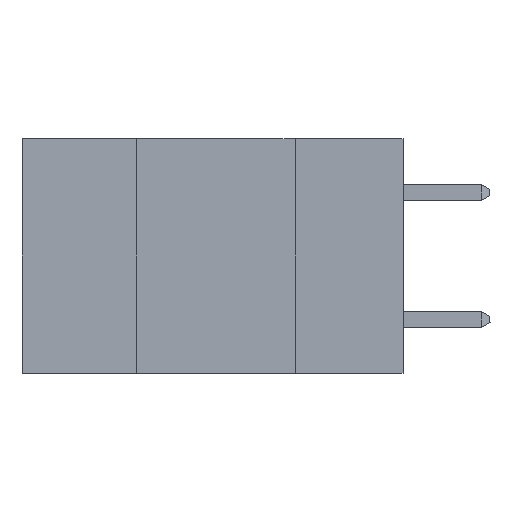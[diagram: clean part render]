
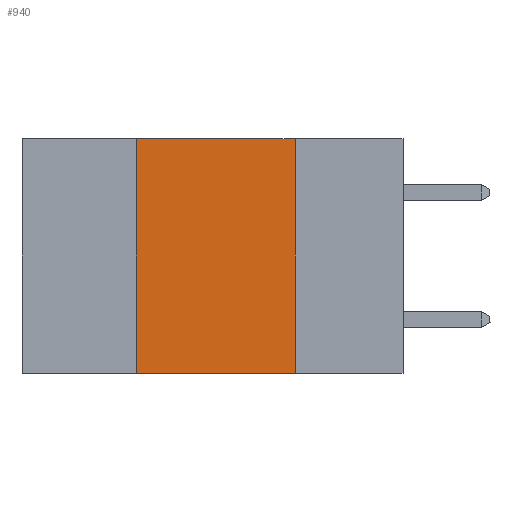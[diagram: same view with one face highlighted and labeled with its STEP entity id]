
A CAD part, left-side view. The second image highlights one B-rep face of the part: STEP entity #940.
In plain terms, the highlighted planar face has unit normal (-1, 0, 0).
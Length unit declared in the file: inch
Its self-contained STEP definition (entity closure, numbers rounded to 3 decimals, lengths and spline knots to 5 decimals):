
#160 = ORIENTED_EDGE ( 'NONE', *, *, #24087, .F. ) ;
#666 = CARTESIAN_POINT ( 'NONE',  ( 0., 0.17, 0. ) ) ;
#940 = ADVANCED_FACE ( 'NONE', ( #27256 ), #1410, .F. ) ;
#1410 = PLANE ( 'NONE',  #10255 ) ;
#1800 = VECTOR ( 'NONE', #24428, 39.37008 ) ;
#1870 = VERTEX_POINT ( 'NONE', #23510 ) ;
#2463 = EDGE_CURVE ( 'NONE', #1870, #14427, #19160, .T. ) ;
#2764 = DIRECTION ( 'NONE',  ( 0., 0., 1. ) ) ;
#2925 = CARTESIAN_POINT ( 'NONE',  ( 0., 0.6, -0.37 ) ) ;
#3157 = LINE ( 'NONE', #17607, #1800 ) ;
#4084 = VECTOR ( 'NONE', #2764, 39.37008 ) ;
#6897 = ORIENTED_EDGE ( 'NONE', *, *, #16684, .F. ) ;
#7790 = ORIENTED_EDGE ( 'NONE', *, *, #2463, .F. ) ;
#9384 = DIRECTION ( 'NONE',  ( 0., -1., 0. ) ) ;
#10255 = AXIS2_PLACEMENT_3D ( 'NONE', #12144, #12056, #14170 ) ;
#10950 = VECTOR ( 'NONE', #19508, 39.37008 ) ;
#11149 = EDGE_LOOP ( 'NONE', ( #6897, #160, #7790, #22038 ) ) ;
#11459 = VECTOR ( 'NONE', #9384, 39.37008 ) ;
#12056 = DIRECTION ( 'NONE',  ( 1., 0., 0. ) ) ;
#12144 = CARTESIAN_POINT ( 'NONE',  ( 0., 0.6, 0. ) ) ;
#13523 = VERTEX_POINT ( 'NONE', #666 ) ;
#13720 = VERTEX_POINT ( 'NONE', #15857 ) ;
#14170 = DIRECTION ( 'NONE',  ( 0., 0., -1. ) ) ;
#14427 = VERTEX_POINT ( 'NONE', #20651 ) ;
#14887 = LINE ( 'NONE', #27289, #10950 ) ;
#15857 = CARTESIAN_POINT ( 'NONE',  ( 0., 0.17, -0.37 ) ) ;
#16684 = EDGE_CURVE ( 'NONE', #13523, #13720, #3157, .T. ) ;
#17238 = CARTESIAN_POINT ( 'NONE',  ( 0., 0.42, 0. ) ) ;
#17607 = CARTESIAN_POINT ( 'NONE',  ( 0., 0.17, 0. ) ) ;
#18461 = LINE ( 'NONE', #2925, #11459 ) ;
#19160 = LINE ( 'NONE', #17238, #4084 ) ;
#19508 = DIRECTION ( 'NONE',  ( 0., -1., 0. ) ) ;
#20651 = CARTESIAN_POINT ( 'NONE',  ( 0., 0.42, 0. ) ) ;
#22038 = ORIENTED_EDGE ( 'NONE', *, *, #27486, .T. ) ;
#23510 = CARTESIAN_POINT ( 'NONE',  ( 0., 0.42, -0.37 ) ) ;
#24087 = EDGE_CURVE ( 'NONE', #14427, #13523, #14887, .T. ) ;
#24428 = DIRECTION ( 'NONE',  ( 0., 0., -1. ) ) ;
#27256 = FACE_OUTER_BOUND ( 'NONE', #11149, .T. ) ;
#27289 = CARTESIAN_POINT ( 'NONE',  ( 0., 0.6, 0. ) ) ;
#27486 = EDGE_CURVE ( 'NONE', #1870, #13720, #18461, .T. ) ;
